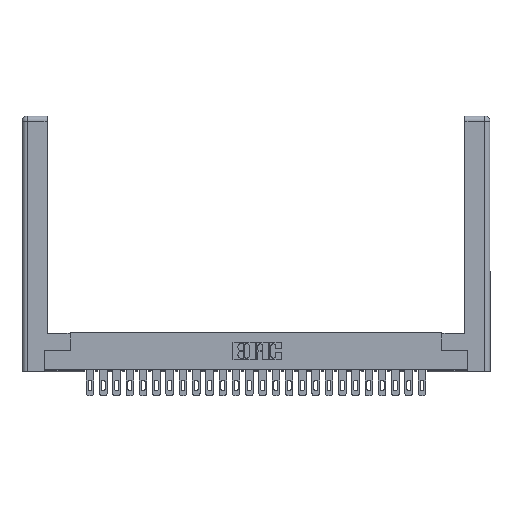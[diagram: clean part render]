
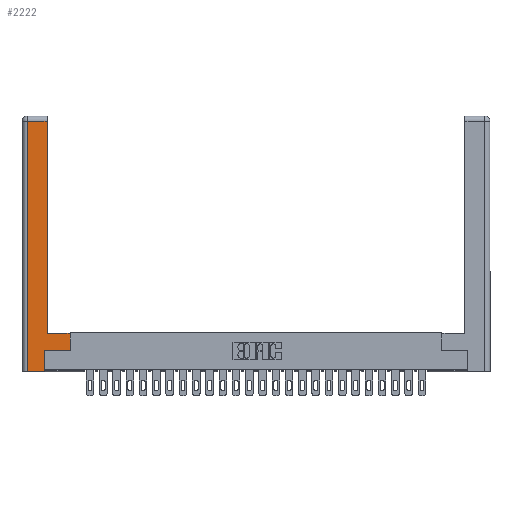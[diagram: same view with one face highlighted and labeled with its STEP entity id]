
A CAD part, top view. The second image highlights one B-rep face of the part: STEP entity #2222.
In plain terms, the highlighted planar face has unit normal (0, 0, 1).
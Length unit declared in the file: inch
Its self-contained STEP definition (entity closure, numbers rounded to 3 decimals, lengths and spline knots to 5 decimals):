
#383 = CARTESIAN_POINT ( 'NONE',  ( 0.295, 3., 0. ) ) ;
#576 = ORIENTED_EDGE ( 'NONE', *, *, #3451, .T. ) ;
#1274 = VERTEX_POINT ( 'NONE', #18121 ) ;
#1451 = LINE ( 'NONE', #25728, #26747 ) ;
#1969 = CARTESIAN_POINT ( 'NONE',  ( 0.0615, 2.94, 0. ) ) ;
#2222 = ADVANCED_FACE ( 'NONE', ( #19664 ), #14125, .F. ) ;
#2415 = LINE ( 'NONE', #1969, #11924 ) ;
#2742 = EDGE_CURVE ( 'NONE', #2932, #7169, #20398, .T. ) ;
#2932 = VERTEX_POINT ( 'NONE', #18806 ) ;
#3451 = EDGE_CURVE ( 'NONE', #19400, #15099, #15255, .T. ) ;
#4978 = ORIENTED_EDGE ( 'NONE', *, *, #8980, .T. ) ;
#7169 = VERTEX_POINT ( 'NONE', #24163 ) ;
#8932 = ORIENTED_EDGE ( 'NONE', *, *, #2742, .T. ) ;
#8980 = EDGE_CURVE ( 'NONE', #11788, #1274, #22201, .T. ) ;
#10719 = CARTESIAN_POINT ( 'NONE',  ( 0.265, 0.245, 0. ) ) ;
#10907 = VECTOR ( 'NONE', #17698, 39.37008 ) ;
#11788 = VERTEX_POINT ( 'NONE', #27042 ) ;
#11924 = VECTOR ( 'NONE', #29664, 39.37008 ) ;
#12367 = CARTESIAN_POINT ( 'NONE',  ( 0.565, 0.245, 0. ) ) ;
#13353 = ORIENTED_EDGE ( 'NONE', *, *, #24928, .T. ) ;
#13655 = DIRECTION ( 'NONE',  ( -1., 0., 0. ) ) ;
#14125 = PLANE ( 'NONE',  #18770 ) ;
#14908 = ORIENTED_EDGE ( 'NONE', *, *, #30326, .T. ) ;
#15078 = CARTESIAN_POINT ( 'NONE',  ( 0.265, 0.245, 0. ) ) ;
#15099 = VERTEX_POINT ( 'NONE', #10719 ) ;
#15255 = LINE ( 'NONE', #15078, #27543 ) ;
#15690 = DIRECTION ( 'NONE',  ( 0., 1., 0. ) ) ;
#16790 = EDGE_CURVE ( 'NONE', #1274, #32677, #2415, .T. ) ;
#17698 = DIRECTION ( 'NONE',  ( 0., 1., 0. ) ) ;
#17732 = DIRECTION ( 'NONE',  ( 0., 1., 0. ) ) ;
#18121 = CARTESIAN_POINT ( 'NONE',  ( 0.295, 2.94, 0. ) ) ;
#18323 = DIRECTION ( 'NONE',  ( 0., -1., 0. ) ) ;
#18768 = VECTOR ( 'NONE', #19860, 39.37008 ) ;
#18770 = AXIS2_PLACEMENT_3D ( 'NONE', #26388, #26510, #28805 ) ;
#18806 = CARTESIAN_POINT ( 'NONE',  ( 0.565, 0.245, 0. ) ) ;
#19400 = VERTEX_POINT ( 'NONE', #20278 ) ;
#19562 = EDGE_CURVE ( 'NONE', #7169, #11788, #31325, .T. ) ;
#19664 = FACE_OUTER_BOUND ( 'NONE', #22794, .T. ) ;
#19860 = DIRECTION ( 'NONE',  ( 1., 0., 0. ) ) ;
#20246 = VECTOR ( 'NONE', #15690, 39.37008 ) ;
#20278 = CARTESIAN_POINT ( 'NONE',  ( 0.265, 0., 0. ) ) ;
#20282 = ORIENTED_EDGE ( 'NONE', *, *, #16790, .T. ) ;
#20398 = LINE ( 'NONE', #32649, #10907 ) ;
#22201 = LINE ( 'NONE', #383, #20246 ) ;
#22653 = VECTOR ( 'NONE', #30327, 39.37008 ) ;
#22794 = EDGE_LOOP ( 'NONE', ( #4978, #20282, #31566, #13353, #576, #14908, #8932, #27768 ) ) ;
#24125 = CARTESIAN_POINT ( 'NONE',  ( 0.295, 0.45, 0. ) ) ;
#24163 = CARTESIAN_POINT ( 'NONE',  ( 0.565, 0.45, 0. ) ) ;
#24892 = CARTESIAN_POINT ( 'NONE',  ( 0.0615, 0., 0. ) ) ;
#24928 = EDGE_CURVE ( 'NONE', #30609, #19400, #29392, .T. ) ;
#25728 = CARTESIAN_POINT ( 'NONE',  ( 0.0615, 0., 0. ) ) ;
#26388 = CARTESIAN_POINT ( 'NONE',  ( 0., 0., 0. ) ) ;
#26510 = DIRECTION ( 'NONE',  ( 0., 0., -1. ) ) ;
#26747 = VECTOR ( 'NONE', #18323, 39.37008 ) ;
#27042 = CARTESIAN_POINT ( 'NONE',  ( 0.295, 0.45, 0. ) ) ;
#27543 = VECTOR ( 'NONE', #17732, 39.37008 ) ;
#27768 = ORIENTED_EDGE ( 'NONE', *, *, #19562, .T. ) ;
#28805 = DIRECTION ( 'NONE',  ( -1., 0., 0. ) ) ;
#28920 = VECTOR ( 'NONE', #13655, 39.37008 ) ;
#29029 = LINE ( 'NONE', #12367, #18768 ) ;
#29392 = LINE ( 'NONE', #30223, #22653 ) ;
#29645 = EDGE_CURVE ( 'NONE', #32677, #30609, #1451, .T. ) ;
#29664 = DIRECTION ( 'NONE',  ( -1., 0., 0. ) ) ;
#30223 = CARTESIAN_POINT ( 'NONE',  ( 0.265, 0., 0. ) ) ;
#30258 = CARTESIAN_POINT ( 'NONE',  ( 0.0615, 2.94, 0. ) ) ;
#30326 = EDGE_CURVE ( 'NONE', #15099, #2932, #29029, .T. ) ;
#30327 = DIRECTION ( 'NONE',  ( 1., 0., 0. ) ) ;
#30609 = VERTEX_POINT ( 'NONE', #24892 ) ;
#31325 = LINE ( 'NONE', #24125, #28920 ) ;
#31566 = ORIENTED_EDGE ( 'NONE', *, *, #29645, .T. ) ;
#32649 = CARTESIAN_POINT ( 'NONE',  ( 0.565, 0.45, 0. ) ) ;
#32677 = VERTEX_POINT ( 'NONE', #30258 ) ;
